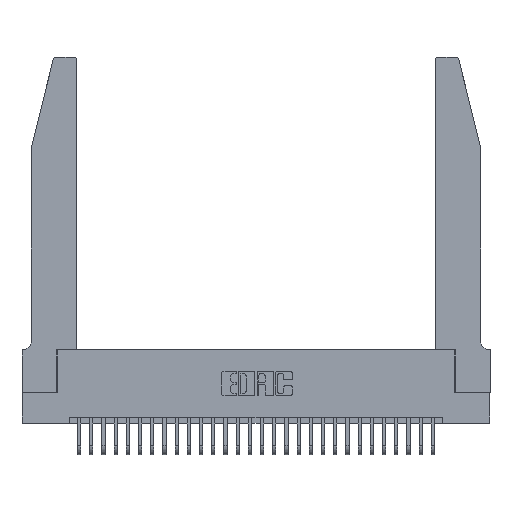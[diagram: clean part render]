
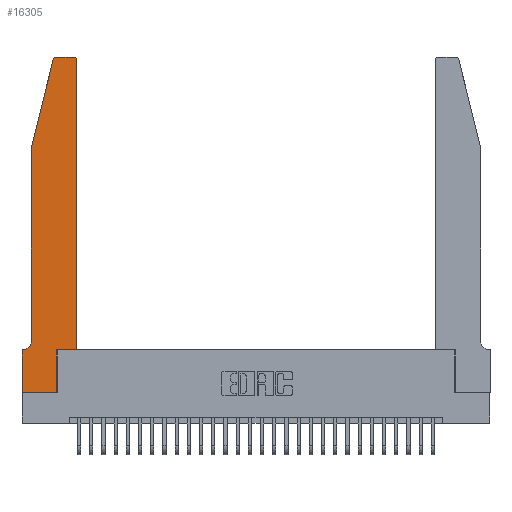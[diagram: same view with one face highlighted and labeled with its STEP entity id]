
A CAD part, top view. The second image highlights one B-rep face of the part: STEP entity #16305.
In plain terms, the highlighted planar face has unit normal (0, 0, 1).
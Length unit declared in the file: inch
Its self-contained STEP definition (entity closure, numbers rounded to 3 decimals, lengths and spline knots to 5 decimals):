
#41 = EDGE_CURVE ( 'NONE', #23968, #13287, #25263, .T. ) ;
#685 = CARTESIAN_POINT ( 'NONE',  ( 0.0755, 2., 0.37 ) ) ;
#1386 = CARTESIAN_POINT ( 'NONE',  ( 0.4205, 2.75, 0.37 ) ) ;
#1695 = ORIENTED_EDGE ( 'NONE', *, *, #14128, .T. ) ;
#2760 = CARTESIAN_POINT ( 'NONE',  ( 0.2605, 2.75, 0.37 ) ) ;
#2825 = DIRECTION ( 'NONE',  ( -0.239, -0.971, 0. ) ) ;
#3493 = CARTESIAN_POINT ( 'NONE',  ( 0.2865, 0.35, 0.37 ) ) ;
#4388 = DIRECTION ( 'NONE',  ( 0., 0., 1. ) ) ;
#4426 = FACE_OUTER_BOUND ( 'NONE', #13056, .T. ) ;
#5258 = VERTEX_POINT ( 'NONE', #15799 ) ;
#5347 = LINE ( 'NONE', #16761, #22399 ) ;
#5492 = DIRECTION ( 'NONE',  ( 0., 0., -1. ) ) ;
#5834 = DIRECTION ( 'NONE',  ( 0., 1., 0. ) ) ;
#6181 = ORIENTED_EDGE ( 'NONE', *, *, #21019, .T. ) ;
#6798 = CARTESIAN_POINT ( 'NONE',  ( 0.284, 2.75, 0.37 ) ) ;
#7004 = DIRECTION ( 'NONE',  ( 0., 0., 1. ) ) ;
#7129 = VECTOR ( 'NONE', #24600, 39.37008 ) ;
#7153 = VECTOR ( 'NONE', #23126, 39.37008 ) ;
#7355 = EDGE_CURVE ( 'NONE', #28817, #9041, #5347, .T. ) ;
#7399 = DIRECTION ( 'NONE',  ( -1., 0., 0. ) ) ;
#7957 = VERTEX_POINT ( 'NONE', #9972 ) ;
#8009 = CARTESIAN_POINT ( 'NONE',  ( 0.284, 2.72, 0.37 ) ) ;
#9041 = VERTEX_POINT ( 'NONE', #9602 ) ;
#9602 = CARTESIAN_POINT ( 'NONE',  ( 0.4505, 0.35, 0.37 ) ) ;
#9900 = CARTESIAN_POINT ( 'NONE',  ( 0., 0., 0.37 ) ) ;
#9911 = DIRECTION ( 'NONE',  ( 0., -1., 0. ) ) ;
#9972 = CARTESIAN_POINT ( 'NONE',  ( 0., 0., 0.37 ) ) ;
#9976 = ORIENTED_EDGE ( 'NONE', *, *, #15505, .T. ) ;
#10038 = ORIENTED_EDGE ( 'NONE', *, *, #41, .T. ) ;
#10274 = DIRECTION ( 'NONE',  ( 1., 0., 0. ) ) ;
#10462 = CARTESIAN_POINT ( 'NONE',  ( 0.0755, 0.42, 0.37 ) ) ;
#10547 = CARTESIAN_POINT ( 'NONE',  ( 0.0755, 0.35, 0.37 ) ) ;
#10672 = EDGE_CURVE ( 'NONE', #14406, #27831, #14655, .T. ) ;
#10751 = CARTESIAN_POINT ( 'NONE',  ( 0.25487, 2.72718, 0.37 ) ) ;
#10793 = ORIENTED_EDGE ( 'NONE', *, *, #21417, .T. ) ;
#11105 = CARTESIAN_POINT ( 'NONE',  ( 0.4505, 2.72, 0.37 ) ) ;
#12376 = VECTOR ( 'NONE', #23823, 39.37008 ) ;
#12401 = AXIS2_PLACEMENT_3D ( 'NONE', #18834, #5492, #21049 ) ;
#12602 = LINE ( 'NONE', #3493, #17768 ) ;
#12707 = VECTOR ( 'NONE', #2825, 39.37008 ) ;
#12781 = VERTEX_POINT ( 'NONE', #6798 ) ;
#12820 = ORIENTED_EDGE ( 'NONE', *, *, #23357, .T. ) ;
#12845 = ORIENTED_EDGE ( 'NONE', *, *, #21172, .T. ) ;
#13056 = EDGE_LOOP ( 'NONE', ( #9976, #1695, #10038, #28798, #24649, #25036, #10793, #6181, #12820, #19691, #12845, #13853 ) ) ;
#13220 = CARTESIAN_POINT ( 'NONE',  ( 0.0755, 2., 0.37 ) ) ;
#13287 = VERTEX_POINT ( 'NONE', #13220 ) ;
#13308 = CARTESIAN_POINT ( 'NONE',  ( 0., 0.35, 0.37 ) ) ;
#13425 = VECTOR ( 'NONE', #26015, 39.37008 ) ;
#13853 = ORIENTED_EDGE ( 'NONE', *, *, #10672, .T. ) ;
#13917 = CARTESIAN_POINT ( 'NONE',  ( 0.0755, 2., 0.37 ) ) ;
#14128 = EDGE_CURVE ( 'NONE', #12781, #23968, #14433, .T. ) ;
#14212 = EDGE_CURVE ( 'NONE', #18894, #19629, #18214, .T. ) ;
#14406 = VERTEX_POINT ( 'NONE', #11105 ) ;
#14433 = CIRCLE ( 'NONE', #22769, 0.03 ) ;
#14655 = CIRCLE ( 'NONE', #22329, 0.03 ) ;
#15505 = EDGE_CURVE ( 'NONE', #27831, #12781, #28596, .T. ) ;
#15799 = CARTESIAN_POINT ( 'NONE',  ( 0.2865, 0., 0.37 ) ) ;
#16305 = ADVANCED_FACE ( 'NONE', ( #4426 ), #26696, .T. ) ;
#16586 = EDGE_CURVE ( 'NONE', #13287, #21205, #20875, .T. ) ;
#16761 = CARTESIAN_POINT ( 'NONE',  ( 0.4505, 0.35, 0.37 ) ) ;
#16793 = VECTOR ( 'NONE', #7399, 39.37008 ) ;
#17324 = CARTESIAN_POINT ( 'NONE',  ( 0.0055, 0.35, 0.37 ) ) ;
#17768 = VECTOR ( 'NONE', #5834, 39.37008 ) ;
#17813 = CARTESIAN_POINT ( 'NONE',  ( 0., 0.35, 0.37 ) ) ;
#18214 = LINE ( 'NONE', #10547, #12376 ) ;
#18834 = CARTESIAN_POINT ( 'NONE',  ( 0.0055, 0.42, 0.37 ) ) ;
#18894 = VERTEX_POINT ( 'NONE', #17324 ) ;
#19227 = CARTESIAN_POINT ( 'NONE',  ( 0.4505, 0.35, 0.37 ) ) ;
#19306 = LINE ( 'NONE', #19227, #13425 ) ;
#19629 = VERTEX_POINT ( 'NONE', #13308 ) ;
#19691 = ORIENTED_EDGE ( 'NONE', *, *, #7355, .T. ) ;
#19998 = DIRECTION ( 'NONE',  ( 1., 0., 0. ) ) ;
#20170 = VECTOR ( 'NONE', #9911, 39.37008 ) ;
#20289 = CARTESIAN_POINT ( 'NONE',  ( 0.4205, 2.72, 0.37 ) ) ;
#20311 = LINE ( 'NONE', #22305, #7129 ) ;
#20780 = CIRCLE ( 'NONE', #12401, 0.07 ) ;
#20875 = LINE ( 'NONE', #685, #20170 ) ;
#21019 = EDGE_CURVE ( 'NONE', #7957, #5258, #24222, .T. ) ;
#21049 = DIRECTION ( 'NONE',  ( -1., 0., 0. ) ) ;
#21172 = EDGE_CURVE ( 'NONE', #9041, #14406, #19306, .T. ) ;
#21205 = VERTEX_POINT ( 'NONE', #10462 ) ;
#21417 = EDGE_CURVE ( 'NONE', #19629, #7957, #20311, .T. ) ;
#22019 = AXIS2_PLACEMENT_3D ( 'NONE', #17813, #4388, #19998 ) ;
#22305 = CARTESIAN_POINT ( 'NONE',  ( 0., 0., 0.37 ) ) ;
#22329 = AXIS2_PLACEMENT_3D ( 'NONE', #20289, #7004, #22543 ) ;
#22399 = VECTOR ( 'NONE', #23343, 39.37008 ) ;
#22543 = DIRECTION ( 'NONE',  ( 1., 0., 0. ) ) ;
#22769 = AXIS2_PLACEMENT_3D ( 'NONE', #8009, #23524, #10274 ) ;
#23126 = DIRECTION ( 'NONE',  ( 1., 0., 0. ) ) ;
#23343 = DIRECTION ( 'NONE',  ( 1., 0., 0. ) ) ;
#23357 = EDGE_CURVE ( 'NONE', #5258, #28817, #12602, .T. ) ;
#23524 = DIRECTION ( 'NONE',  ( 0., 0., 1. ) ) ;
#23823 = DIRECTION ( 'NONE',  ( -1., 0., 0. ) ) ;
#23968 = VERTEX_POINT ( 'NONE', #10751 ) ;
#24222 = LINE ( 'NONE', #9900, #7153 ) ;
#24600 = DIRECTION ( 'NONE',  ( 0., -1., 0. ) ) ;
#24649 = ORIENTED_EDGE ( 'NONE', *, *, #25588, .T. ) ;
#25036 = ORIENTED_EDGE ( 'NONE', *, *, #14212, .T. ) ;
#25263 = LINE ( 'NONE', #13917, #12707 ) ;
#25588 = EDGE_CURVE ( 'NONE', #21205, #18894, #20780, .T. ) ;
#26015 = DIRECTION ( 'NONE',  ( 0., 1., 0. ) ) ;
#26696 = PLANE ( 'NONE',  #22019 ) ;
#27801 = CARTESIAN_POINT ( 'NONE',  ( 0.2865, 0.35, 0.37 ) ) ;
#27831 = VERTEX_POINT ( 'NONE', #1386 ) ;
#28596 = LINE ( 'NONE', #2760, #16793 ) ;
#28798 = ORIENTED_EDGE ( 'NONE', *, *, #16586, .T. ) ;
#28817 = VERTEX_POINT ( 'NONE', #27801 ) ;
